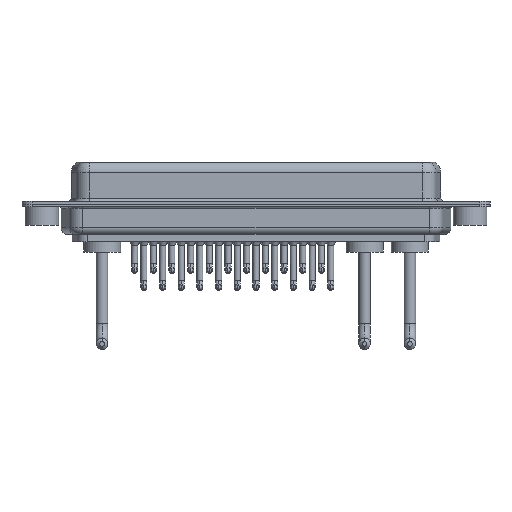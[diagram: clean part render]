
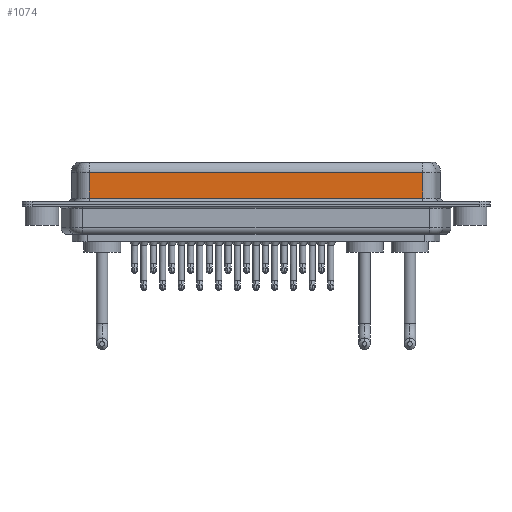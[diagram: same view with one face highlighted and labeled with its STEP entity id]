
A CAD part, front view. The second image highlights one B-rep face of the part: STEP entity #1074.
In plain terms, the highlighted planar face has unit normal (0, -1, 0).
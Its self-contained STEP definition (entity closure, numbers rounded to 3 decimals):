
#27 = VERTEX_POINT ( 'NONE', #8556 ) ;
#129 = CARTESIAN_POINT ( 'NONE',  ( 56.462, -3.95, 4.65 ) ) ;
#1074 = ADVANCED_FACE ( 'NONE', ( #23138 ), #11899, .F. ) ;
#1112 = DIRECTION ( 'NONE',  ( 1., 0., 0. ) ) ;
#1239 = VECTOR ( 'NONE', #10996, 1000. ) ;
#1491 = DIRECTION ( 'NONE',  ( 0., 0., -1. ) ) ;
#1683 = VERTEX_POINT ( 'NONE', #10540 ) ;
#2503 = ORIENTED_EDGE ( 'NONE', *, *, #10866, .T. ) ;
#3533 = CARTESIAN_POINT ( 'NONE',  ( 7.038, -3.95, 6.4 ) ) ;
#6800 = ORIENTED_EDGE ( 'NONE', *, *, #10970, .T. ) ;
#8556 = CARTESIAN_POINT ( 'NONE',  ( 7.038, -3.95, 0.9 ) ) ;
#9646 = VECTOR ( 'NONE', #20428, 1000. ) ;
#10207 = DIRECTION ( 'NONE',  ( 0., 0., 1. ) ) ;
#10540 = CARTESIAN_POINT ( 'NONE',  ( 7.038, -3.95, 4.65 ) ) ;
#10758 = CARTESIAN_POINT ( 'NONE',  ( 56.462, -3.95, 0.9 ) ) ;
#10866 = EDGE_CURVE ( 'NONE', #27, #16227, #14135, .T. ) ;
#10874 = CARTESIAN_POINT ( 'NONE',  ( 56.462, -3.95, 6.4 ) ) ;
#10970 = EDGE_CURVE ( 'NONE', #14263, #1683, #12801, .T. ) ;
#10996 = DIRECTION ( 'NONE',  ( -1., 0., 0. ) ) ;
#11899 = PLANE ( 'NONE',  #18667 ) ;
#12409 = VECTOR ( 'NONE', #1112, 1000. ) ;
#12801 = LINE ( 'NONE', #129, #1239 ) ;
#13105 = EDGE_CURVE ( 'NONE', #1683, #27, #16321, .T. ) ;
#14135 = LINE ( 'NONE', #10758, #12409 ) ;
#14263 = VERTEX_POINT ( 'NONE', #19253 ) ;
#14484 = LINE ( 'NONE', #10874, #9646 ) ;
#15098 = ORIENTED_EDGE ( 'NONE', *, *, #13105, .T. ) ;
#15783 = ORIENTED_EDGE ( 'NONE', *, *, #20043, .F. ) ;
#16227 = VERTEX_POINT ( 'NONE', #20083 ) ;
#16321 = LINE ( 'NONE', #3533, #23296 ) ;
#17567 = DIRECTION ( 'NONE',  ( 0., 1., 0. ) ) ;
#18667 = AXIS2_PLACEMENT_3D ( 'NONE', #21342, #17567, #10207 ) ;
#19253 = CARTESIAN_POINT ( 'NONE',  ( 56.462, -3.95, 4.65 ) ) ;
#20043 = EDGE_CURVE ( 'NONE', #14263, #16227, #14484, .T. ) ;
#20083 = CARTESIAN_POINT ( 'NONE',  ( 56.462, -3.95, 0.9 ) ) ;
#20428 = DIRECTION ( 'NONE',  ( 0., 0., -1. ) ) ;
#21342 = CARTESIAN_POINT ( 'NONE',  ( 56.462, -3.95, 6.4 ) ) ;
#22905 = EDGE_LOOP ( 'NONE', ( #15783, #6800, #15098, #2503 ) ) ;
#23138 = FACE_OUTER_BOUND ( 'NONE', #22905, .T. ) ;
#23296 = VECTOR ( 'NONE', #1491, 1000. ) ;
